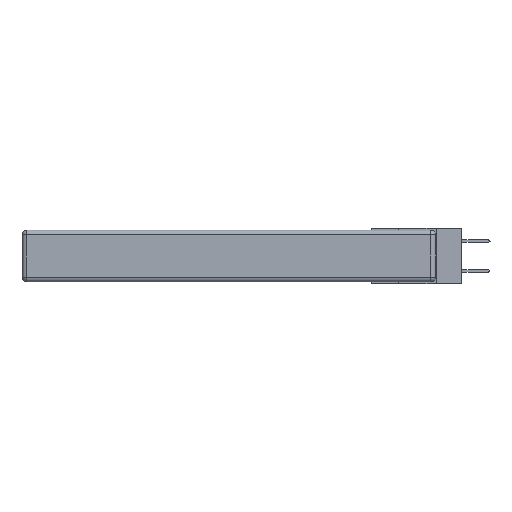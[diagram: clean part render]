
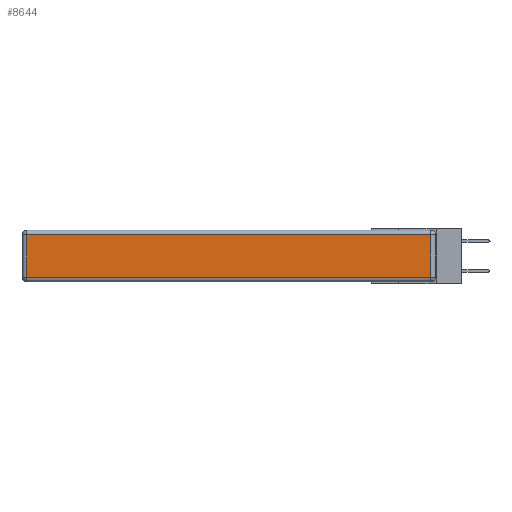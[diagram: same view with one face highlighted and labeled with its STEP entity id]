
A CAD part, left-side view. The second image highlights one B-rep face of the part: STEP entity #8644.
In plain terms, the highlighted planar face has unit normal (-1, 0, 0).
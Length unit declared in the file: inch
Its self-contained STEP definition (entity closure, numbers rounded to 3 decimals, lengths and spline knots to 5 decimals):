
#227 = CARTESIAN_POINT ( 'NONE',  ( 0., 2.72, -0.343 ) ) ;
#254 = ORIENTED_EDGE ( 'NONE', *, *, #5965, .T. ) ;
#432 = EDGE_CURVE ( 'NONE', #7111, #7277, #3924, .T. ) ;
#916 = ORIENTED_EDGE ( 'NONE', *, *, #8344, .T. ) ;
#1361 = AXIS2_PLACEMENT_3D ( 'NONE', #13122, #7831, #6702 ) ;
#1557 = ORIENTED_EDGE ( 'NONE', *, *, #432, .T. ) ;
#2613 = CARTESIAN_POINT ( 'NONE',  ( 0., 0.03, -0.03 ) ) ;
#2720 = PLANE ( 'NONE',  #1361 ) ;
#2951 = VERTEX_POINT ( 'NONE', #9521 ) ;
#3045 = DIRECTION ( 'NONE',  ( 0., 1., 0. ) ) ;
#3412 = DIRECTION ( 'NONE',  ( 0., 0., -1. ) ) ;
#3924 = LINE ( 'NONE', #6674, #10022 ) ;
#4273 = VECTOR ( 'NONE', #3045, 39.37008 ) ;
#5268 = FACE_OUTER_BOUND ( 'NONE', #7890, .T. ) ;
#5965 = EDGE_CURVE ( 'NONE', #2951, #8776, #6459, .T. ) ;
#6459 = LINE ( 'NONE', #227, #12588 ) ;
#6674 = CARTESIAN_POINT ( 'NONE',  ( 0., 0.03, -0.343 ) ) ;
#6702 = DIRECTION ( 'NONE',  ( 0., 0., 1. ) ) ;
#6890 = LINE ( 'NONE', #11327, #4273 ) ;
#7111 = VERTEX_POINT ( 'NONE', #12042 ) ;
#7277 = VERTEX_POINT ( 'NONE', #2613 ) ;
#7428 = CARTESIAN_POINT ( 'NONE',  ( 0., 0., -0.313 ) ) ;
#7831 = DIRECTION ( 'NONE',  ( -1., 0., 0. ) ) ;
#7890 = EDGE_LOOP ( 'NONE', ( #916, #1557, #10390, #254 ) ) ;
#8344 = EDGE_CURVE ( 'NONE', #8776, #7111, #11695, .T. ) ;
#8644 = ADVANCED_FACE ( 'NONE', ( #5268 ), #2720, .T. ) ;
#8776 = VERTEX_POINT ( 'NONE', #13509 ) ;
#9361 = DIRECTION ( 'NONE',  ( 0., -1., 0. ) ) ;
#9521 = CARTESIAN_POINT ( 'NONE',  ( 0., 2.72, -0.03 ) ) ;
#10022 = VECTOR ( 'NONE', #13095, 39.37008 ) ;
#10390 = ORIENTED_EDGE ( 'NONE', *, *, #11330, .T. ) ;
#10531 = VECTOR ( 'NONE', #9361, 39.37008 ) ;
#11327 = CARTESIAN_POINT ( 'NONE',  ( 0., 2.75, -0.03 ) ) ;
#11330 = EDGE_CURVE ( 'NONE', #7277, #2951, #6890, .T. ) ;
#11695 = LINE ( 'NONE', #7428, #10531 ) ;
#12042 = CARTESIAN_POINT ( 'NONE',  ( 0., 0.03, -0.313 ) ) ;
#12588 = VECTOR ( 'NONE', #3412, 39.37008 ) ;
#13095 = DIRECTION ( 'NONE',  ( 0., 0., 1. ) ) ;
#13122 = CARTESIAN_POINT ( 'NONE',  ( 0., 0., -0.343 ) ) ;
#13509 = CARTESIAN_POINT ( 'NONE',  ( 0., 2.72, -0.313 ) ) ;
